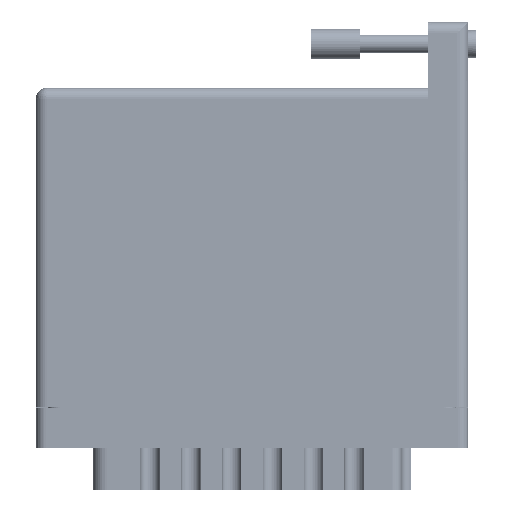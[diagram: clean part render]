
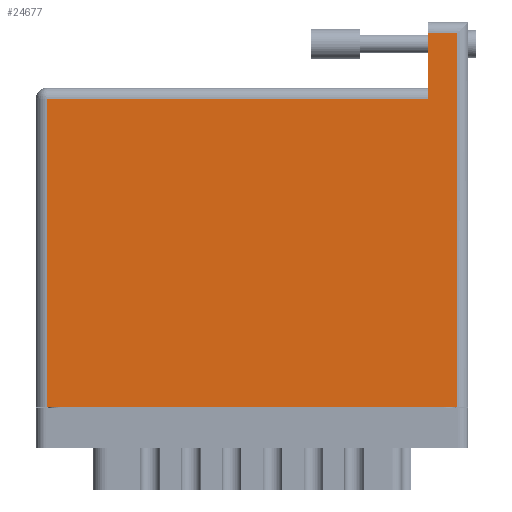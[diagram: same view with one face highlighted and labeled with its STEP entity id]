
A CAD part, front view. The second image highlights one B-rep face of the part: STEP entity #24677.
In plain terms, the highlighted face is planar.
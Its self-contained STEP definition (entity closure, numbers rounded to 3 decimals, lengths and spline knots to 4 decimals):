
#1033 = ORIENTED_EDGE ( 'NONE', *, *, #85954, .T. ) ;
#3194 = CARTESIAN_POINT ( 'NONE',  ( 2.499, 2.38, 0. ) ) ;
#10647 = CARTESIAN_POINT ( 'NONE',  ( 2.685, 0., 0. ) ) ;
#11196 = VERTEX_POINT ( 'NONE', #30595 ) ;
#12079 = VERTEX_POINT ( 'NONE', #3194 ) ;
#17913 = ORIENTED_EDGE ( 'NONE', *, *, #61101, .T. ) ;
#21064 = CARTESIAN_POINT ( 'NONE',  ( 0., 2.03, 0. ) ) ;
#21322 = DIRECTION ( 'NONE',  ( 1., 0., 0. ) ) ;
#21396 = VECTOR ( 'NONE', #84124, 39.3701 ) ;
#21437 = VECTOR ( 'NONE', #59242, 39.3701 ) ;
#21785 = LINE ( 'NONE', #61413, #35655 ) ;
#23896 = ORIENTED_EDGE ( 'NONE', *, *, #70356, .T. ) ;
#24677 = ADVANCED_FACE ( 'NONE', ( #31167 ), #95614, .F. ) ;
#26042 = ORIENTED_EDGE ( 'NONE', *, *, #30442, .T. ) ;
#28525 = DIRECTION ( 'NONE',  ( -1., 0., 0. ) ) ;
#29123 = LINE ( 'NONE', #55701, #66391 ) ;
#30442 = EDGE_CURVE ( 'NONE', #85506, #11196, #57990, .T. ) ;
#30595 = CARTESIAN_POINT ( 'NONE',  ( 0.07, 0., 0. ) ) ;
#30994 = EDGE_LOOP ( 'NONE', ( #68250, #23896, #26042, #1033, #54133, #17913 ) ) ;
#31167 = FACE_OUTER_BOUND ( 'NONE', #30994, .T. ) ;
#35655 = VECTOR ( 'NONE', #54883, 39.3701 ) ;
#36362 = DIRECTION ( 'NONE',  ( 0., -1., 0. ) ) ;
#37316 = CARTESIAN_POINT ( 'NONE',  ( 0.07, 0., 0. ) ) ;
#38526 = VERTEX_POINT ( 'NONE', #45890 ) ;
#38758 = VERTEX_POINT ( 'NONE', #47794 ) ;
#43942 = VECTOR ( 'NONE', #21322, 39.3701 ) ;
#45390 = AXIS2_PLACEMENT_3D ( 'NONE', #21064, #50296, #28525 ) ;
#45859 = LINE ( 'NONE', #51403, #21437 ) ;
#45890 = CARTESIAN_POINT ( 'NONE',  ( 2.499, 1.96, 0. ) ) ;
#47794 = CARTESIAN_POINT ( 'NONE',  ( 2.685, 2.38, 0. ) ) ;
#48827 = DIRECTION ( 'NONE',  ( 0., 1., 0. ) ) ;
#50296 = DIRECTION ( 'NONE',  ( 0., 0., -1. ) ) ;
#51403 = CARTESIAN_POINT ( 'NONE',  ( 2.499, 2.45, 0. ) ) ;
#54133 = ORIENTED_EDGE ( 'NONE', *, *, #92859, .T. ) ;
#54883 = DIRECTION ( 'NONE',  ( -1., 0., 0. ) ) ;
#55701 = CARTESIAN_POINT ( 'NONE',  ( 2.685, 2.45, 0. ) ) ;
#56673 = EDGE_CURVE ( 'NONE', #12079, #38526, #45859, .T. ) ;
#57764 = CARTESIAN_POINT ( 'NONE',  ( 0., 0., 0. ) ) ;
#57990 = LINE ( 'NONE', #37316, #90476 ) ;
#59242 = DIRECTION ( 'NONE',  ( 0., -1., 0. ) ) ;
#61101 = EDGE_CURVE ( 'NONE', #38758, #12079, #21785, .T. ) ;
#61413 = CARTESIAN_POINT ( 'NONE',  ( 0., 2.38, 0. ) ) ;
#66391 = VECTOR ( 'NONE', #48827, 39.3701 ) ;
#67602 = CARTESIAN_POINT ( 'NONE',  ( 0.07, 1.96, 0. ) ) ;
#68250 = ORIENTED_EDGE ( 'NONE', *, *, #56673, .T. ) ;
#68538 = CARTESIAN_POINT ( 'NONE',  ( 0., 1.96, 0. ) ) ;
#70356 = EDGE_CURVE ( 'NONE', #38526, #85506, #71422, .T. ) ;
#71422 = LINE ( 'NONE', #68538, #21396 ) ;
#73766 = VERTEX_POINT ( 'NONE', #10647 ) ;
#77659 = LINE ( 'NONE', #57764, #43942 ) ;
#84124 = DIRECTION ( 'NONE',  ( -1., 0., 0. ) ) ;
#85506 = VERTEX_POINT ( 'NONE', #67602 ) ;
#85954 = EDGE_CURVE ( 'NONE', #11196, #73766, #77659, .T. ) ;
#90476 = VECTOR ( 'NONE', #36362, 39.3701 ) ;
#92859 = EDGE_CURVE ( 'NONE', #73766, #38758, #29123, .T. ) ;
#95614 = PLANE ( 'NONE',  #45390 ) ;
